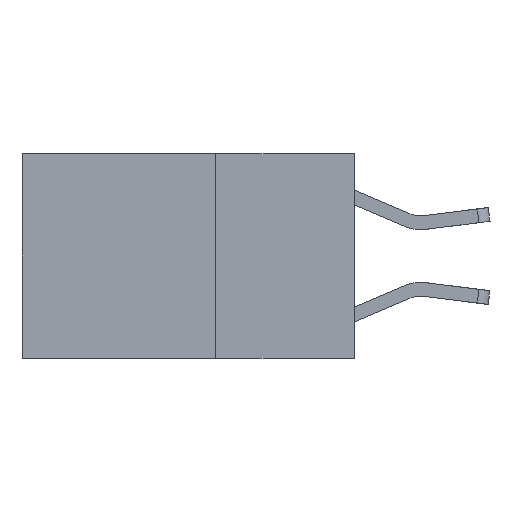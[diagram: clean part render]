
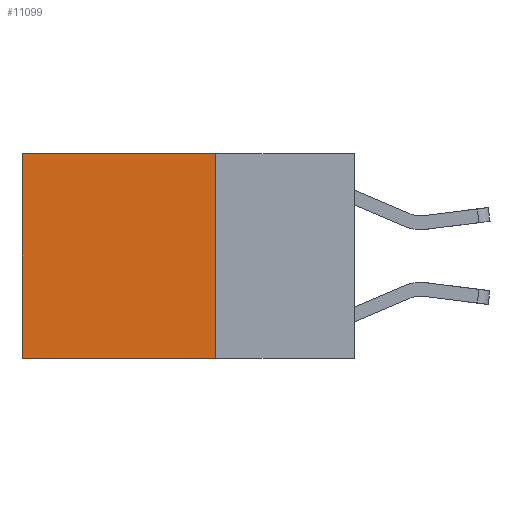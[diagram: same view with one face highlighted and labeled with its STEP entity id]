
A CAD part, left-side view. The second image highlights one B-rep face of the part: STEP entity #11099.
In plain terms, the highlighted planar face has unit normal (-1, 0, 0).
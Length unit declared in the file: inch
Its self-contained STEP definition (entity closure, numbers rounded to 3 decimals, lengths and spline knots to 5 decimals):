
#3 = AXIS2_PLACEMENT_3D ( 'NONE', #11325, #9512, #3931 ) ;
#97 = LINE ( 'NONE', #7085, #11895 ) ;
#346 = VERTEX_POINT ( 'NONE', #11082 ) ;
#467 = EDGE_CURVE ( 'NONE', #346, #8142, #515, .T. ) ;
#515 = LINE ( 'NONE', #6612, #2741 ) ;
#1307 = FACE_OUTER_BOUND ( 'NONE', #8358, .T. ) ;
#2178 = CARTESIAN_POINT ( 'NONE',  ( 0.2625, 0.25, 0. ) ) ;
#2469 = VERTEX_POINT ( 'NONE', #2178 ) ;
#2741 = VECTOR ( 'NONE', #10332, 39.37008 ) ;
#2749 = CARTESIAN_POINT ( 'NONE',  ( 0.2625, 0.25, 0. ) ) ;
#2875 = EDGE_CURVE ( 'NONE', #2469, #346, #6624, .T. ) ;
#3296 = ORIENTED_EDGE ( 'NONE', *, *, #2875, .T. ) ;
#3566 = CARTESIAN_POINT ( 'NONE',  ( 0.2625, 0.6, -0.37 ) ) ;
#3931 = DIRECTION ( 'NONE',  ( 0., 0., -1. ) ) ;
#4701 = EDGE_CURVE ( 'NONE', #5778, #8142, #5466, .T. ) ;
#5397 = ORIENTED_EDGE ( 'NONE', *, *, #11694, .F. ) ;
#5466 = LINE ( 'NONE', #6913, #10455 ) ;
#5778 = VERTEX_POINT ( 'NONE', #6538 ) ;
#6538 = CARTESIAN_POINT ( 'NONE',  ( 0.2625, 0.25, -0.37 ) ) ;
#6612 = CARTESIAN_POINT ( 'NONE',  ( 0.2625, 0.6, 0. ) ) ;
#6624 = LINE ( 'NONE', #2749, #11276 ) ;
#6913 = CARTESIAN_POINT ( 'NONE',  ( 0.2625, 0.25, -0.37 ) ) ;
#6958 = ORIENTED_EDGE ( 'NONE', *, *, #4701, .F. ) ;
#7085 = CARTESIAN_POINT ( 'NONE',  ( 0.2625, 0.25, 0. ) ) ;
#8019 = DIRECTION ( 'NONE',  ( 0., 0., -1. ) ) ;
#8142 = VERTEX_POINT ( 'NONE', #3566 ) ;
#8358 = EDGE_LOOP ( 'NONE', ( #11898, #6958, #5397, #3296 ) ) ;
#8769 = DIRECTION ( 'NONE',  ( 0., 1., 0. ) ) ;
#9251 = DIRECTION ( 'NONE',  ( 0., 1., 0. ) ) ;
#9512 = DIRECTION ( 'NONE',  ( 1., 0., 0. ) ) ;
#10332 = DIRECTION ( 'NONE',  ( 0., 0., -1. ) ) ;
#10408 = PLANE ( 'NONE',  #3 ) ;
#10455 = VECTOR ( 'NONE', #8769, 39.37008 ) ;
#11082 = CARTESIAN_POINT ( 'NONE',  ( 0.2625, 0.6, 0. ) ) ;
#11099 = ADVANCED_FACE ( 'NONE', ( #1307 ), #10408, .F. ) ;
#11276 = VECTOR ( 'NONE', #9251, 39.37008 ) ;
#11325 = CARTESIAN_POINT ( 'NONE',  ( 0.2625, 0.25, 0. ) ) ;
#11694 = EDGE_CURVE ( 'NONE', #2469, #5778, #97, .T. ) ;
#11895 = VECTOR ( 'NONE', #8019, 39.37008 ) ;
#11898 = ORIENTED_EDGE ( 'NONE', *, *, #467, .T. ) ;
